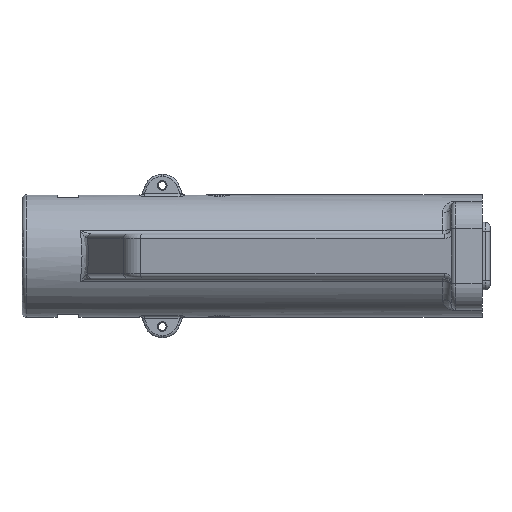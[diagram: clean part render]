
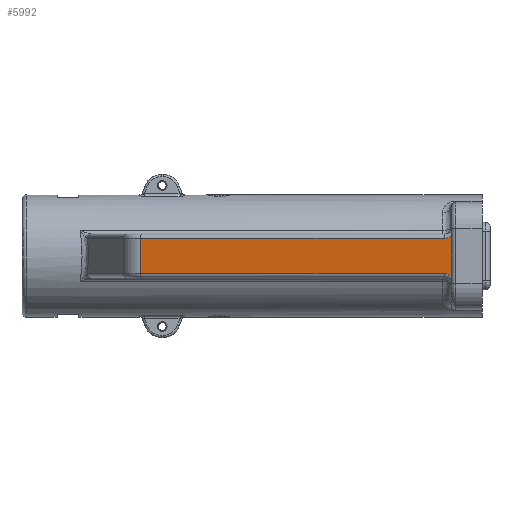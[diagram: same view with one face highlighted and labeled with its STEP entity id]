
A CAD part, front view. The second image highlights one B-rep face of the part: STEP entity #5992.
In plain terms, the highlighted planar face has unit normal (-0.147, -0.989, 0).
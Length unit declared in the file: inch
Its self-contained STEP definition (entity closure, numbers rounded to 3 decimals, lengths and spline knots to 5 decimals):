
#139=PLANE('',#6745);
#192=ELLIPSE('',#6491,0.12637,0.125);
#194=ELLIPSE('',#6494,0.12637,0.125);
#329=LINE('',#10334,#691);
#353=LINE('',#10427,#715);
#419=LINE('',#11284,#781);
#466=LINE('',#11567,#828);
#691=VECTOR('',#7245,0.3937);
#715=VECTOR('',#7315,0.05);
#781=VECTOR('',#7693,0.3937);
#828=VECTOR('',#7918,0.05);
#1483=FACE_OUTER_BOUND('',#1871,.T.);
#1871=EDGE_LOOP('',(#5501,#5502,#5503,#5504,#5505,#5506));
#2580=VERTEX_POINT('',#10317);
#2583=VERTEX_POINT('',#10325);
#2626=VERTEX_POINT('',#10426);
#2642=VERTEX_POINT('',#10643);
#2728=VERTEX_POINT('',#11282);
#2760=VERTEX_POINT('',#11562);
#3202=EDGE_CURVE('',#2580,#2583,#329,.T.);
#3246=EDGE_CURVE('',#2583,#2626,#353,.T.);
#3428=EDGE_CURVE('',#2728,#2642,#419,.T.);
#3512=EDGE_CURVE('',#2642,#2760,#192,.T.);
#3514=EDGE_CURVE('',#2760,#2580,#466,.T.);
#3516=EDGE_CURVE('',#2626,#2728,#194,.T.);
#5501=ORIENTED_EDGE('',*,*,#3202,.F.);
#5502=ORIENTED_EDGE('',*,*,#3514,.F.);
#5503=ORIENTED_EDGE('',*,*,#3512,.F.);
#5504=ORIENTED_EDGE('',*,*,#3428,.F.);
#5505=ORIENTED_EDGE('',*,*,#3516,.F.);
#5506=ORIENTED_EDGE('',*,*,#3246,.F.);
#5992=ADVANCED_FACE('',(#1483),#139,.T.);
#6491=AXIS2_PLACEMENT_3D('',#11564,#7913,#7914);
#6494=AXIS2_PLACEMENT_3D('',#11594,#7921,#7922);
#6745=AXIS2_PLACEMENT_3D('',#12360,#8552,#8553);
#7245=DIRECTION('',(0.,0.,1.));
#7315=DIRECTION('',(0.989,-0.147,0.));
#7693=DIRECTION('',(0.,0.,-1.));
#7913=DIRECTION('center_axis',(-0.147,-0.989,0.));
#7914=DIRECTION('ref_axis',(0.989,-0.147,0.));
#7918=DIRECTION('',(-0.989,0.147,0.));
#7921=DIRECTION('center_axis',(-0.147,-0.989,0.));
#7922=DIRECTION('ref_axis',(0.989,-0.147,0.));
#8552=DIRECTION('center_axis',(-0.147,-0.989,0.));
#8553=DIRECTION('ref_axis',(0.989,-0.147,0.));
#10317=CARTESIAN_POINT('',(2.6544,-2.27295,-0.2));
#10325=CARTESIAN_POINT('',(2.6544,-2.27295,0.2));
#10334=CARTESIAN_POINT('',(2.6544,-2.27295,0.));
#10426=CARTESIAN_POINT('',(6.11765,-2.78776,0.2));
#10427=CARTESIAN_POINT('',(3.24535,-2.36079,0.2));
#10643=CARTESIAN_POINT('',(6.2,-2.8,-0.23096));
#11282=CARTESIAN_POINT('',(6.2,-2.8,0.23096));
#11284=CARTESIAN_POINT('',(6.2,-2.8,0.));
#11562=CARTESIAN_POINT('',(6.11765,-2.78776,-0.2));
#11564=CARTESIAN_POINT('Origin',(6.11765,-2.78776,-0.325));
#11567=CARTESIAN_POINT('',(3.24535,-2.36079,-0.2));
#11594=CARTESIAN_POINT('Origin',(6.11765,-2.78776,0.325));
#12360=CARTESIAN_POINT('Origin',(2.5,-2.25,0.));
